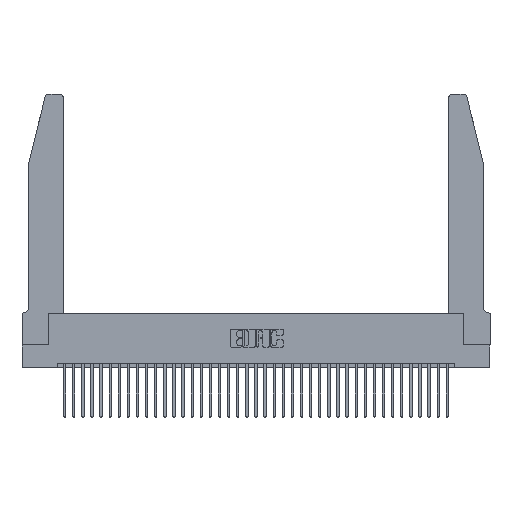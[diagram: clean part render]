
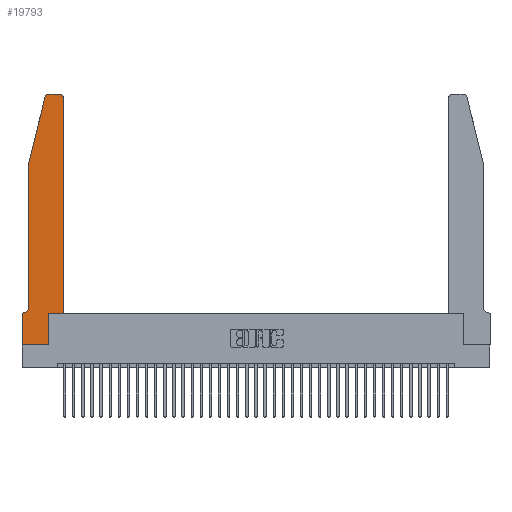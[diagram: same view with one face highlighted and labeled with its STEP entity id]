
A CAD part, top view. The second image highlights one B-rep face of the part: STEP entity #19793.
In plain terms, the highlighted planar face has unit normal (0, 0, 1).
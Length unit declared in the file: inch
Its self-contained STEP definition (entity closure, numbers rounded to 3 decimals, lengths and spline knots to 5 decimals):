
#325 = VECTOR ( 'NONE', #28374, 39.37008 ) ;
#694 = LINE ( 'NONE', #3701, #28992 ) ;
#1224 = VECTOR ( 'NONE', #17941, 39.37008 ) ;
#1240 = ORIENTED_EDGE ( 'NONE', *, *, #29523, .T. ) ;
#2036 = CARTESIAN_POINT ( 'NONE',  ( 0.4505, 0.35, 0.37 ) ) ;
#2191 = EDGE_CURVE ( 'NONE', #24705, #32565, #29785, .T. ) ;
#2592 = VECTOR ( 'NONE', #18594, 39.37008 ) ;
#2648 = DIRECTION ( 'NONE',  ( 1., 0., 0. ) ) ;
#2918 = AXIS2_PLACEMENT_3D ( 'NONE', #32216, #20673, #5960 ) ;
#3701 = CARTESIAN_POINT ( 'NONE',  ( 0., 0., 0.37 ) ) ;
#3815 = ORIENTED_EDGE ( 'NONE', *, *, #11374, .T. ) ;
#3834 = DIRECTION ( 'NONE',  ( 0., 1., 0. ) ) ;
#3960 = VERTEX_POINT ( 'NONE', #32244 ) ;
#4096 = CARTESIAN_POINT ( 'NONE',  ( 0.4205, 2.72, 0.37 ) ) ;
#4464 = EDGE_CURVE ( 'NONE', #3960, #22879, #13370, .T. ) ;
#5442 = ORIENTED_EDGE ( 'NONE', *, *, #28788, .T. ) ;
#5960 = DIRECTION ( 'NONE',  ( 1., 0., 0. ) ) ;
#6206 = CARTESIAN_POINT ( 'NONE',  ( 0.4505, 0.35, 0.37 ) ) ;
#6285 = EDGE_CURVE ( 'NONE', #17913, #8623, #11865, .T. ) ;
#6560 = EDGE_LOOP ( 'NONE', ( #3815, #33407, #15705, #7313, #13040, #8924, #14403, #14981, #21746, #1240, #5442, #23383 ) ) ;
#6567 = DIRECTION ( 'NONE',  ( 0., 0., 1. ) ) ;
#7313 = ORIENTED_EDGE ( 'NONE', *, *, #11604, .T. ) ;
#7375 = DIRECTION ( 'NONE',  ( -1., 0., 0. ) ) ;
#7480 = EDGE_CURVE ( 'NONE', #22879, #29431, #27604, .T. ) ;
#7723 = DIRECTION ( 'NONE',  ( -1., 0., 0. ) ) ;
#7787 = CARTESIAN_POINT ( 'NONE',  ( 0., 0.35, 0.37 ) ) ;
#7973 = CARTESIAN_POINT ( 'NONE',  ( 0.0755, 2., 0.37 ) ) ;
#8240 = EDGE_CURVE ( 'NONE', #19117, #24705, #21986, .T. ) ;
#8350 = DIRECTION ( 'NONE',  ( -1., 0., 0. ) ) ;
#8531 = CIRCLE ( 'NONE', #19313, 0.03 ) ;
#8623 = VERTEX_POINT ( 'NONE', #21201 ) ;
#8924 = ORIENTED_EDGE ( 'NONE', *, *, #2191, .T. ) ;
#10737 = DIRECTION ( 'NONE',  ( -0.239, -0.971, 0. ) ) ;
#11374 = EDGE_CURVE ( 'NONE', #18057, #3960, #21729, .T. ) ;
#11604 = EDGE_CURVE ( 'NONE', #29431, #19117, #32347, .T. ) ;
#11865 = LINE ( 'NONE', #27554, #2592 ) ;
#12371 = CARTESIAN_POINT ( 'NONE',  ( 0.2865, 0.35, 0.37 ) ) ;
#13040 = ORIENTED_EDGE ( 'NONE', *, *, #8240, .T. ) ;
#13370 = CIRCLE ( 'NONE', #2918, 0.03 ) ;
#13732 = LINE ( 'NONE', #6206, #1224 ) ;
#14403 = ORIENTED_EDGE ( 'NONE', *, *, #25083, .T. ) ;
#14512 = VECTOR ( 'NONE', #8350, 39.37008 ) ;
#14981 = ORIENTED_EDGE ( 'NONE', *, *, #6285, .T. ) ;
#15392 = CARTESIAN_POINT ( 'NONE',  ( 0., 0., 0.37 ) ) ;
#15488 = DIRECTION ( 'NONE',  ( 1., 0., 0. ) ) ;
#15637 = AXIS2_PLACEMENT_3D ( 'NONE', #16500, #31427, #7723 ) ;
#15705 = ORIENTED_EDGE ( 'NONE', *, *, #7480, .T. ) ;
#15736 = CARTESIAN_POINT ( 'NONE',  ( 0.4205, 2.75, 0.37 ) ) ;
#16466 = VECTOR ( 'NONE', #10737, 39.37008 ) ;
#16500 = CARTESIAN_POINT ( 'NONE',  ( 0.0055, 0.42, 0.37 ) ) ;
#17042 = CARTESIAN_POINT ( 'NONE',  ( 0.0755, 0.42, 0.37 ) ) ;
#17673 = VERTEX_POINT ( 'NONE', #36704 ) ;
#17913 = VERTEX_POINT ( 'NONE', #15392 ) ;
#17941 = DIRECTION ( 'NONE',  ( 1., 0., 0. ) ) ;
#18048 = VECTOR ( 'NONE', #3834, 39.37008 ) ;
#18057 = VERTEX_POINT ( 'NONE', #15736 ) ;
#18594 = DIRECTION ( 'NONE',  ( 1., 0., 0. ) ) ;
#18822 = DIRECTION ( 'NONE',  ( 0., -1., 0. ) ) ;
#19117 = VERTEX_POINT ( 'NONE', #17042 ) ;
#19313 = AXIS2_PLACEMENT_3D ( 'NONE', #4096, #6567, #15488 ) ;
#19530 = CARTESIAN_POINT ( 'NONE',  ( 0.4505, 0.35, 0.37 ) ) ;
#19793 = ADVANCED_FACE ( 'NONE', ( #31661 ), #35251, .T. ) ;
#20097 = CARTESIAN_POINT ( 'NONE',  ( 0., 0.35, 0.37 ) ) ;
#20673 = DIRECTION ( 'NONE',  ( 0., 0., 1. ) ) ;
#21201 = CARTESIAN_POINT ( 'NONE',  ( 0.2865, 0., 0.37 ) ) ;
#21729 = LINE ( 'NONE', #24950, #24022 ) ;
#21746 = ORIENTED_EDGE ( 'NONE', *, *, #35805, .T. ) ;
#21986 = CIRCLE ( 'NONE', #15637, 0.07 ) ;
#22350 = CARTESIAN_POINT ( 'NONE',  ( 0.0055, 0.35, 0.37 ) ) ;
#22879 = VERTEX_POINT ( 'NONE', #32109 ) ;
#23383 = ORIENTED_EDGE ( 'NONE', *, *, #33563, .T. ) ;
#23751 = VERTEX_POINT ( 'NONE', #36016 ) ;
#24022 = VECTOR ( 'NONE', #7375, 39.37008 ) ;
#24705 = VERTEX_POINT ( 'NONE', #22350 ) ;
#24950 = CARTESIAN_POINT ( 'NONE',  ( 0.2605, 2.75, 0.37 ) ) ;
#25083 = EDGE_CURVE ( 'NONE', #32565, #17913, #694, .T. ) ;
#25578 = AXIS2_PLACEMENT_3D ( 'NONE', #20097, #26199, #2648 ) ;
#26199 = DIRECTION ( 'NONE',  ( 0., 0., 1. ) ) ;
#27309 = VECTOR ( 'NONE', #32061, 39.37008 ) ;
#27554 = CARTESIAN_POINT ( 'NONE',  ( 0., 0., 0.37 ) ) ;
#27604 = LINE ( 'NONE', #31606, #16466 ) ;
#28374 = DIRECTION ( 'NONE',  ( 0., 1., 0. ) ) ;
#28788 = EDGE_CURVE ( 'NONE', #33177, #23751, #29078, .T. ) ;
#28992 = VECTOR ( 'NONE', #18822, 39.37008 ) ;
#29078 = LINE ( 'NONE', #19530, #325 ) ;
#29205 = CARTESIAN_POINT ( 'NONE',  ( 0.0755, 0.35, 0.37 ) ) ;
#29431 = VERTEX_POINT ( 'NONE', #7973 ) ;
#29523 = EDGE_CURVE ( 'NONE', #17673, #33177, #13732, .T. ) ;
#29785 = LINE ( 'NONE', #29205, #14512 ) ;
#31427 = DIRECTION ( 'NONE',  ( 0., 0., -1. ) ) ;
#31606 = CARTESIAN_POINT ( 'NONE',  ( 0.0755, 2., 0.37 ) ) ;
#31661 = FACE_OUTER_BOUND ( 'NONE', #6560, .T. ) ;
#32061 = DIRECTION ( 'NONE',  ( 0., -1., 0. ) ) ;
#32109 = CARTESIAN_POINT ( 'NONE',  ( 0.25487, 2.72718, 0.37 ) ) ;
#32216 = CARTESIAN_POINT ( 'NONE',  ( 0.284, 2.72, 0.37 ) ) ;
#32244 = CARTESIAN_POINT ( 'NONE',  ( 0.284, 2.75, 0.37 ) ) ;
#32302 = CARTESIAN_POINT ( 'NONE',  ( 0.0755, 2., 0.37 ) ) ;
#32347 = LINE ( 'NONE', #32302, #27309 ) ;
#32565 = VERTEX_POINT ( 'NONE', #7787 ) ;
#33177 = VERTEX_POINT ( 'NONE', #2036 ) ;
#33407 = ORIENTED_EDGE ( 'NONE', *, *, #4464, .T. ) ;
#33563 = EDGE_CURVE ( 'NONE', #23751, #18057, #8531, .T. ) ;
#33835 = LINE ( 'NONE', #12371, #18048 ) ;
#35251 = PLANE ( 'NONE',  #25578 ) ;
#35805 = EDGE_CURVE ( 'NONE', #8623, #17673, #33835, .T. ) ;
#36016 = CARTESIAN_POINT ( 'NONE',  ( 0.4505, 2.72, 0.37 ) ) ;
#36704 = CARTESIAN_POINT ( 'NONE',  ( 0.2865, 0.35, 0.37 ) ) ;
